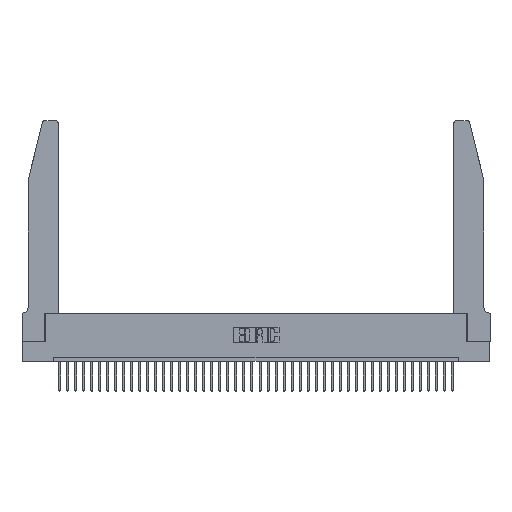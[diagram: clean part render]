
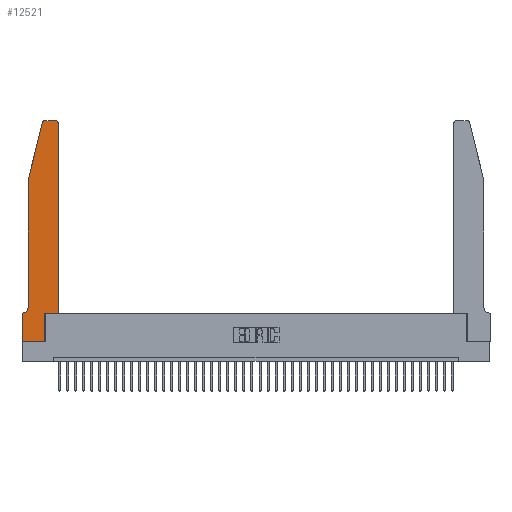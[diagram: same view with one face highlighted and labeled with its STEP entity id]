
A CAD part, top view. The second image highlights one B-rep face of the part: STEP entity #12521.
In plain terms, the highlighted planar face has unit normal (0, 0, 1).
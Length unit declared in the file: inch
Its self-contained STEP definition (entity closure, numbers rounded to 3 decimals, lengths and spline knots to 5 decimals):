
#103 = LINE ( 'NONE', #2353, #8624 ) ;
#146 = EDGE_LOOP ( 'NONE', ( #21620, #35245, #6047, #3065, #1860, #31759, #26948, #35829, #12339, #33690, #28237, #390 ) ) ;
#390 = ORIENTED_EDGE ( 'NONE', *, *, #39939, .T. ) ;
#448 = CARTESIAN_POINT ( 'NONE',  ( 0.4505, 2.72, 0.37 ) ) ;
#713 = VERTEX_POINT ( 'NONE', #38644 ) ;
#987 = CARTESIAN_POINT ( 'NONE',  ( 0.4505, 0.35, 0.37 ) ) ;
#1075 = DIRECTION ( 'NONE',  ( -1., 0., 0. ) ) ;
#1557 = PLANE ( 'NONE',  #26194 ) ;
#1686 = DIRECTION ( 'NONE',  ( 0., 0., -1. ) ) ;
#1860 = ORIENTED_EDGE ( 'NONE', *, *, #29356, .T. ) ;
#2353 = CARTESIAN_POINT ( 'NONE',  ( 0.0755, 2., 0.37 ) ) ;
#2632 = DIRECTION ( 'NONE',  ( 0., 0., 1. ) ) ;
#3065 = ORIENTED_EDGE ( 'NONE', *, *, #32421, .T. ) ;
#3830 = VERTEX_POINT ( 'NONE', #987 ) ;
#4475 = CARTESIAN_POINT ( 'NONE',  ( 0.284, 2.75, 0.37 ) ) ;
#5162 = DIRECTION ( 'NONE',  ( 0., -1., 0. ) ) ;
#5573 = DIRECTION ( 'NONE',  ( 0., 0., 1. ) ) ;
#5762 = CARTESIAN_POINT ( 'NONE',  ( 0.2605, 2.75, 0.37 ) ) ;
#6047 = ORIENTED_EDGE ( 'NONE', *, *, #27348, .T. ) ;
#6079 = CIRCLE ( 'NONE', #23398, 0.03 ) ;
#6354 = EDGE_CURVE ( 'NONE', #19666, #23731, #23834, .T. ) ;
#7138 = CIRCLE ( 'NONE', #16844, 0.03 ) ;
#7999 = DIRECTION ( 'NONE',  ( 0., 0., 1. ) ) ;
#8354 = DIRECTION ( 'NONE',  ( 1., 0., 0. ) ) ;
#8520 = EDGE_CURVE ( 'NONE', #23731, #38683, #16595, .T. ) ;
#8624 = VECTOR ( 'NONE', #5162, 39.37008 ) ;
#8788 = DIRECTION ( 'NONE',  ( 0., 1., 0. ) ) ;
#9293 = VERTEX_POINT ( 'NONE', #27520 ) ;
#10372 = LINE ( 'NONE', #10641, #39315 ) ;
#10458 = DIRECTION ( 'NONE',  ( 1., 0., 0. ) ) ;
#10641 = CARTESIAN_POINT ( 'NONE',  ( 0.4505, 0.35, 0.37 ) ) ;
#10725 = CARTESIAN_POINT ( 'NONE',  ( 0.0055, 0.42, 0.37 ) ) ;
#10897 = CARTESIAN_POINT ( 'NONE',  ( 0., 0., 0.37 ) ) ;
#11040 = DIRECTION ( 'NONE',  ( -0.239, -0.971, 0. ) ) ;
#11714 = DIRECTION ( 'NONE',  ( 1., 0., 0. ) ) ;
#12051 = DIRECTION ( 'NONE',  ( -1., 0., 0. ) ) ;
#12315 = DIRECTION ( 'NONE',  ( 1., 0., 0. ) ) ;
#12339 = ORIENTED_EDGE ( 'NONE', *, *, #33158, .T. ) ;
#12521 = ADVANCED_FACE ( 'NONE', ( #14862 ), #1557, .T. ) ;
#12549 = LINE ( 'NONE', #24978, #34523 ) ;
#12818 = VERTEX_POINT ( 'NONE', #4475 ) ;
#13304 = VECTOR ( 'NONE', #30978, 39.37008 ) ;
#13308 = VECTOR ( 'NONE', #25970, 39.37008 ) ;
#13692 = CARTESIAN_POINT ( 'NONE',  ( 0.4505, 0.35, 0.37 ) ) ;
#14862 = FACE_OUTER_BOUND ( 'NONE', #146, .T. ) ;
#14871 = VECTOR ( 'NONE', #12051, 39.37008 ) ;
#14988 = CARTESIAN_POINT ( 'NONE',  ( 0.4205, 2.75, 0.37 ) ) ;
#16254 = CARTESIAN_POINT ( 'NONE',  ( 0.0755, 0.35, 0.37 ) ) ;
#16595 = LINE ( 'NONE', #30548, #17664 ) ;
#16844 = AXIS2_PLACEMENT_3D ( 'NONE', #25133, #2632, #12315 ) ;
#17664 = VECTOR ( 'NONE', #8354, 39.37008 ) ;
#18263 = EDGE_CURVE ( 'NONE', #12818, #9293, #7138, .T. ) ;
#18362 = VERTEX_POINT ( 'NONE', #14988 ) ;
#19348 = LINE ( 'NONE', #5762, #14871 ) ;
#19666 = VERTEX_POINT ( 'NONE', #19995 ) ;
#19995 = CARTESIAN_POINT ( 'NONE',  ( 0., 0.35, 0.37 ) ) ;
#20000 = DIRECTION ( 'NONE',  ( 0., 1., 0. ) ) ;
#20846 = CARTESIAN_POINT ( 'NONE',  ( 0.0755, 2., 0.37 ) ) ;
#21620 = ORIENTED_EDGE ( 'NONE', *, *, #36180, .T. ) ;
#23056 = DIRECTION ( 'NONE',  ( -1., 0., 0. ) ) ;
#23398 = AXIS2_PLACEMENT_3D ( 'NONE', #34308, #5573, #11714 ) ;
#23626 = LINE ( 'NONE', #20846, #31167 ) ;
#23731 = VERTEX_POINT ( 'NONE', #10897 ) ;
#23834 = LINE ( 'NONE', #30689, #13304 ) ;
#23901 = CIRCLE ( 'NONE', #34252, 0.07 ) ;
#24601 = LINE ( 'NONE', #16254, #32463 ) ;
#24827 = VERTEX_POINT ( 'NONE', #30452 ) ;
#24978 = CARTESIAN_POINT ( 'NONE',  ( 0.2865, 0.35, 0.37 ) ) ;
#25133 = CARTESIAN_POINT ( 'NONE',  ( 0.284, 2.72, 0.37 ) ) ;
#25229 = VERTEX_POINT ( 'NONE', #32711 ) ;
#25572 = VERTEX_POINT ( 'NONE', #448 ) ;
#25970 = DIRECTION ( 'NONE',  ( 1., 0., 0. ) ) ;
#26194 = AXIS2_PLACEMENT_3D ( 'NONE', #27105, #7999, #10458 ) ;
#26948 = ORIENTED_EDGE ( 'NONE', *, *, #6354, .T. ) ;
#27105 = CARTESIAN_POINT ( 'NONE',  ( 0., 0.35, 0.37 ) ) ;
#27348 = EDGE_CURVE ( 'NONE', #9293, #713, #23626, .T. ) ;
#27520 = CARTESIAN_POINT ( 'NONE',  ( 0.25487, 2.72718, 0.37 ) ) ;
#27836 = LINE ( 'NONE', #13692, #13308 ) ;
#28004 = CARTESIAN_POINT ( 'NONE',  ( 0.0055, 0.35, 0.37 ) ) ;
#28140 = CARTESIAN_POINT ( 'NONE',  ( 0.2865, 0., 0.37 ) ) ;
#28237 = ORIENTED_EDGE ( 'NONE', *, *, #35213, .T. ) ;
#28239 = EDGE_CURVE ( 'NONE', #28306, #19666, #24601, .T. ) ;
#28306 = VERTEX_POINT ( 'NONE', #28004 ) ;
#29356 = EDGE_CURVE ( 'NONE', #25229, #28306, #23901, .T. ) ;
#30452 = CARTESIAN_POINT ( 'NONE',  ( 0.2865, 0.35, 0.37 ) ) ;
#30548 = CARTESIAN_POINT ( 'NONE',  ( 0., 0., 0.37 ) ) ;
#30689 = CARTESIAN_POINT ( 'NONE',  ( 0., 0., 0.37 ) ) ;
#30978 = DIRECTION ( 'NONE',  ( 0., -1., 0. ) ) ;
#31167 = VECTOR ( 'NONE', #11040, 39.37008 ) ;
#31759 = ORIENTED_EDGE ( 'NONE', *, *, #28239, .T. ) ;
#32421 = EDGE_CURVE ( 'NONE', #713, #25229, #103, .T. ) ;
#32463 = VECTOR ( 'NONE', #23056, 39.37008 ) ;
#32711 = CARTESIAN_POINT ( 'NONE',  ( 0.0755, 0.42, 0.37 ) ) ;
#33158 = EDGE_CURVE ( 'NONE', #38683, #24827, #12549, .T. ) ;
#33690 = ORIENTED_EDGE ( 'NONE', *, *, #36919, .T. ) ;
#34252 = AXIS2_PLACEMENT_3D ( 'NONE', #10725, #1686, #1075 ) ;
#34308 = CARTESIAN_POINT ( 'NONE',  ( 0.4205, 2.72, 0.37 ) ) ;
#34523 = VECTOR ( 'NONE', #8788, 39.37008 ) ;
#35213 = EDGE_CURVE ( 'NONE', #3830, #25572, #10372, .T. ) ;
#35245 = ORIENTED_EDGE ( 'NONE', *, *, #18263, .T. ) ;
#35829 = ORIENTED_EDGE ( 'NONE', *, *, #8520, .T. ) ;
#36180 = EDGE_CURVE ( 'NONE', #18362, #12818, #19348, .T. ) ;
#36919 = EDGE_CURVE ( 'NONE', #24827, #3830, #27836, .T. ) ;
#38644 = CARTESIAN_POINT ( 'NONE',  ( 0.0755, 2., 0.37 ) ) ;
#38683 = VERTEX_POINT ( 'NONE', #28140 ) ;
#39315 = VECTOR ( 'NONE', #20000, 39.37008 ) ;
#39939 = EDGE_CURVE ( 'NONE', #25572, #18362, #6079, .T. ) ;
